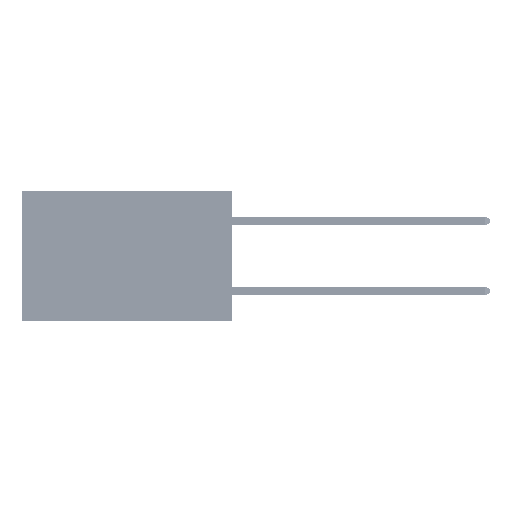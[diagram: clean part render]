
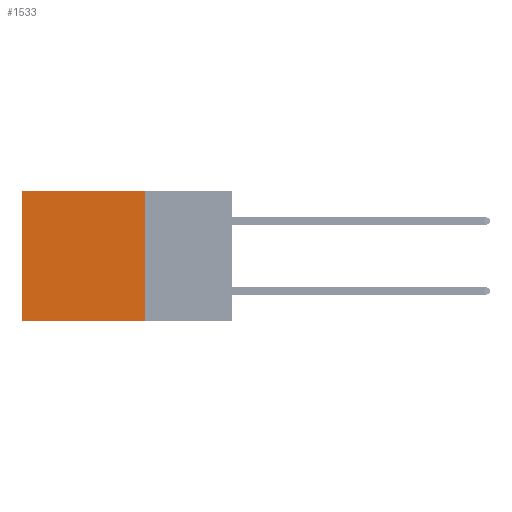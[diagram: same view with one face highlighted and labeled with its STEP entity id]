
A CAD part, left-side view. The second image highlights one B-rep face of the part: STEP entity #1533.
In plain terms, the highlighted planar face has unit normal (-1, 0, 0).
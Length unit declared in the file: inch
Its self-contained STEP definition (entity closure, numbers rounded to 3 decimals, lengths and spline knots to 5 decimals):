
#616 = CARTESIAN_POINT ( 'NONE',  ( 0.2875, 0.6, 0. ) ) ;
#1349 = EDGE_CURVE ( 'NONE', #30460, #3043, #47561, .T. ) ;
#1533 = ADVANCED_FACE ( 'NONE', ( #19217 ), #6065, .F. ) ;
#1653 = LINE ( 'NONE', #45038, #29796 ) ;
#3043 = VERTEX_POINT ( 'NONE', #40489 ) ;
#6065 = PLANE ( 'NONE',  #47444 ) ;
#7552 = CARTESIAN_POINT ( 'NONE',  ( 0.2875, 0.25, -0.37 ) ) ;
#7650 = EDGE_LOOP ( 'NONE', ( #34502, #43268, #38374, #32053 ) ) ;
#8882 = DIRECTION ( 'NONE',  ( 0., 1., 0. ) ) ;
#9881 = DIRECTION ( 'NONE',  ( 1., 0., 0. ) ) ;
#11473 = CARTESIAN_POINT ( 'NONE',  ( 0.2875, 0.25, 0. ) ) ;
#11918 = VECTOR ( 'NONE', #34288, 39.37008 ) ;
#12394 = LINE ( 'NONE', #616, #31503 ) ;
#12399 = EDGE_CURVE ( 'NONE', #36175, #30460, #1653, .T. ) ;
#13082 = LINE ( 'NONE', #11473, #11918 ) ;
#17414 = VECTOR ( 'NONE', #8882, 39.37008 ) ;
#19217 = FACE_OUTER_BOUND ( 'NONE', #7650, .T. ) ;
#21831 = CARTESIAN_POINT ( 'NONE',  ( 0.2875, 0.6, 0. ) ) ;
#22956 = CARTESIAN_POINT ( 'NONE',  ( 0.2875, 0.25, 0. ) ) ;
#29796 = VECTOR ( 'NONE', #33931, 39.37008 ) ;
#30460 = VERTEX_POINT ( 'NONE', #7552 ) ;
#31503 = VECTOR ( 'NONE', #46119, 39.37008 ) ;
#32053 = ORIENTED_EDGE ( 'NONE', *, *, #32954, .T. ) ;
#32954 = EDGE_CURVE ( 'NONE', #36175, #35437, #13082, .T. ) ;
#33931 = DIRECTION ( 'NONE',  ( 0., 0., -1. ) ) ;
#34288 = DIRECTION ( 'NONE',  ( 0., 1., 0. ) ) ;
#34502 = ORIENTED_EDGE ( 'NONE', *, *, #48075, .T. ) ;
#35437 = VERTEX_POINT ( 'NONE', #21831 ) ;
#36175 = VERTEX_POINT ( 'NONE', #22956 ) ;
#36506 = DIRECTION ( 'NONE',  ( 0., 0., -1. ) ) ;
#38374 = ORIENTED_EDGE ( 'NONE', *, *, #12399, .F. ) ;
#40489 = CARTESIAN_POINT ( 'NONE',  ( 0.2875, 0.6, -0.37 ) ) ;
#42890 = CARTESIAN_POINT ( 'NONE',  ( 0.2875, 0.25, -0.37 ) ) ;
#43268 = ORIENTED_EDGE ( 'NONE', *, *, #1349, .F. ) ;
#45038 = CARTESIAN_POINT ( 'NONE',  ( 0.2875, 0.25, 0. ) ) ;
#46119 = DIRECTION ( 'NONE',  ( 0., 0., -1. ) ) ;
#47444 = AXIS2_PLACEMENT_3D ( 'NONE', #47641, #9881, #36506 ) ;
#47561 = LINE ( 'NONE', #42890, #17414 ) ;
#47641 = CARTESIAN_POINT ( 'NONE',  ( 0.2875, 0.25, 0. ) ) ;
#48075 = EDGE_CURVE ( 'NONE', #35437, #3043, #12394, .T. ) ;
